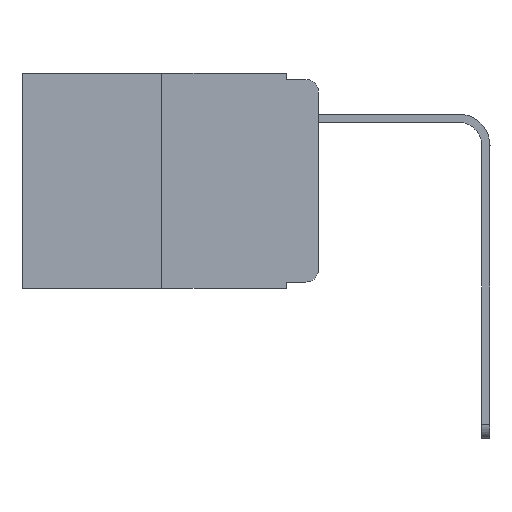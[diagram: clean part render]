
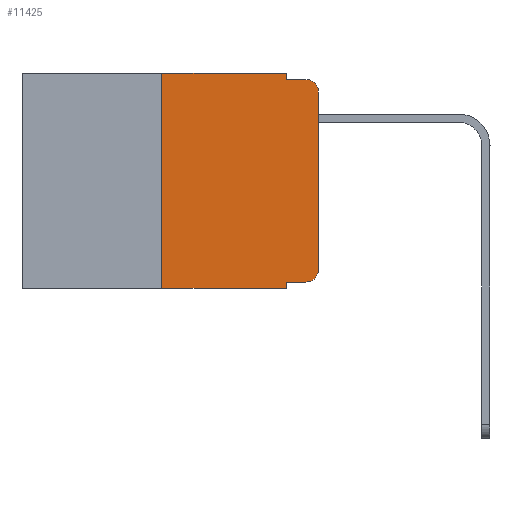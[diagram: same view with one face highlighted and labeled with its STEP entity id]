
A CAD part, left-side view. The second image highlights one B-rep face of the part: STEP entity #11425.
In plain terms, the highlighted planar face has unit normal (-1, 0, 0).
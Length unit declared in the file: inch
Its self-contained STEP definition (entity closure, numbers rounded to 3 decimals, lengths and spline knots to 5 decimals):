
#719 = VECTOR ( 'NONE', #6921, 39.37008 ) ;
#738 = CIRCLE ( 'NONE', #8596, 0.02 ) ;
#768 = DIRECTION ( 'NONE',  ( 1., 0., 0. ) ) ;
#1142 = CARTESIAN_POINT ( 'NONE',  ( 0., 0.051, -0.333 ) ) ;
#1463 = CARTESIAN_POINT ( 'NONE',  ( 0., 0.051, 0. ) ) ;
#1573 = VECTOR ( 'NONE', #10688, 39.37008 ) ;
#1905 = ORIENTED_EDGE ( 'NONE', *, *, #14306, .F. ) ;
#2020 = CARTESIAN_POINT ( 'NONE',  ( 0., 0.051, -0.343 ) ) ;
#2275 = LINE ( 'NONE', #13349, #10521 ) ;
#2339 = CARTESIAN_POINT ( 'NONE',  ( 0., 0., 0. ) ) ;
#2434 = EDGE_CURVE ( 'NONE', #6077, #4303, #13875, .T. ) ;
#2493 = DIRECTION ( 'NONE',  ( 0., -1., 0. ) ) ;
#2670 = EDGE_CURVE ( 'NONE', #12390, #6077, #7057, .T. ) ;
#2777 = CARTESIAN_POINT ( 'NONE',  ( 0., 0.25, 0. ) ) ;
#2807 = CARTESIAN_POINT ( 'NONE',  ( 0., 0.25, 0. ) ) ;
#2841 = ORIENTED_EDGE ( 'NONE', *, *, #4128, .T. ) ;
#2845 = EDGE_CURVE ( 'NONE', #5202, #4857, #7710, .T. ) ;
#2945 = ORIENTED_EDGE ( 'NONE', *, *, #12953, .T. ) ;
#3243 = ORIENTED_EDGE ( 'NONE', *, *, #2845, .F. ) ;
#3553 = CIRCLE ( 'NONE', #8118, 0.02 ) ;
#3591 = CARTESIAN_POINT ( 'NONE',  ( 0., 0.473, -0.343 ) ) ;
#3606 = VECTOR ( 'NONE', #11554, 39.37008 ) ;
#3711 = ORIENTED_EDGE ( 'NONE', *, *, #2434, .F. ) ;
#3738 = DIRECTION ( 'NONE',  ( 0., -1., 0. ) ) ;
#3807 = VERTEX_POINT ( 'NONE', #2020 ) ;
#3950 = VERTEX_POINT ( 'NONE', #11435 ) ;
#4086 = VECTOR ( 'NONE', #3738, 39.37008 ) ;
#4126 = CARTESIAN_POINT ( 'NONE',  ( 0., 0.473, 0. ) ) ;
#4128 = EDGE_CURVE ( 'NONE', #10105, #5263, #7349, .T. ) ;
#4303 = VERTEX_POINT ( 'NONE', #12466 ) ;
#4337 = CARTESIAN_POINT ( 'NONE',  ( 0., 0.02, -0.03 ) ) ;
#4547 = ORIENTED_EDGE ( 'NONE', *, *, #9594, .T. ) ;
#4581 = CARTESIAN_POINT ( 'NONE',  ( 0., 0.051, -0.01 ) ) ;
#4683 = DIRECTION ( 'NONE',  ( 0., -1., 0. ) ) ;
#4857 = VERTEX_POINT ( 'NONE', #2777 ) ;
#5202 = VERTEX_POINT ( 'NONE', #13880 ) ;
#5263 = VERTEX_POINT ( 'NONE', #11961 ) ;
#5633 = ORIENTED_EDGE ( 'NONE', *, *, #11027, .T. ) ;
#6077 = VERTEX_POINT ( 'NONE', #4581 ) ;
#6212 = LINE ( 'NONE', #3591, #7928 ) ;
#6633 = DIRECTION ( 'NONE',  ( 0., 0., -1. ) ) ;
#6648 = CARTESIAN_POINT ( 'NONE',  ( 0., 0.051, -0.333 ) ) ;
#6921 = DIRECTION ( 'NONE',  ( 0., 0., -1. ) ) ;
#7057 = LINE ( 'NONE', #12367, #719 ) ;
#7072 = VECTOR ( 'NONE', #2493, 39.37008 ) ;
#7349 = LINE ( 'NONE', #1142, #10670 ) ;
#7529 = ORIENTED_EDGE ( 'NONE', *, *, #13094, .F. ) ;
#7585 = DIRECTION ( 'NONE',  ( 0., 0., -1. ) ) ;
#7710 = LINE ( 'NONE', #2807, #1573 ) ;
#7928 = VECTOR ( 'NONE', #4683, 39.37008 ) ;
#8118 = AXIS2_PLACEMENT_3D ( 'NONE', #4337, #12115, #7585 ) ;
#8596 = AXIS2_PLACEMENT_3D ( 'NONE', #12585, #13663, #11418 ) ;
#9594 = EDGE_CURVE ( 'NONE', #11531, #3950, #9907, .T. ) ;
#9907 = LINE ( 'NONE', #2339, #3606 ) ;
#9993 = EDGE_LOOP ( 'NONE', ( #4547, #5633, #3711, #12923, #7529, #3243, #2945, #1905, #2841, #13363 ) ) ;
#10105 = VERTEX_POINT ( 'NONE', #6648 ) ;
#10115 = AXIS2_PLACEMENT_3D ( 'NONE', #4126, #768, #14008 ) ;
#10212 = DIRECTION ( 'NONE',  ( 0., -1., 0. ) ) ;
#10442 = CARTESIAN_POINT ( 'NONE',  ( 0., 0.051, -0.01 ) ) ;
#10521 = VECTOR ( 'NONE', #6633, 39.37008 ) ;
#10619 = PLANE ( 'NONE',  #10115 ) ;
#10670 = VECTOR ( 'NONE', #10212, 39.37008 ) ;
#10688 = DIRECTION ( 'NONE',  ( 0., 0., 1. ) ) ;
#10802 = EDGE_CURVE ( 'NONE', #5263, #11531, #738, .T. ) ;
#11027 = EDGE_CURVE ( 'NONE', #3950, #4303, #3553, .T. ) ;
#11417 = FACE_OUTER_BOUND ( 'NONE', #9993, .T. ) ;
#11418 = DIRECTION ( 'NONE',  ( 0., 0., -1. ) ) ;
#11425 = ADVANCED_FACE ( 'NONE', ( #11417 ), #10619, .F. ) ;
#11435 = CARTESIAN_POINT ( 'NONE',  ( 0., 0., -0.03 ) ) ;
#11531 = VERTEX_POINT ( 'NONE', #12919 ) ;
#11554 = DIRECTION ( 'NONE',  ( 0., 0., 1. ) ) ;
#11961 = CARTESIAN_POINT ( 'NONE',  ( 0., 0.02, -0.333 ) ) ;
#12115 = DIRECTION ( 'NONE',  ( -1., 0., 0. ) ) ;
#12367 = CARTESIAN_POINT ( 'NONE',  ( 0., 0.051, 0. ) ) ;
#12390 = VERTEX_POINT ( 'NONE', #1463 ) ;
#12466 = CARTESIAN_POINT ( 'NONE',  ( 0., 0.02, -0.01 ) ) ;
#12585 = CARTESIAN_POINT ( 'NONE',  ( 0., 0.02, -0.313 ) ) ;
#12779 = CARTESIAN_POINT ( 'NONE',  ( 0., 0.473, 0. ) ) ;
#12919 = CARTESIAN_POINT ( 'NONE',  ( 0., 0., -0.313 ) ) ;
#12923 = ORIENTED_EDGE ( 'NONE', *, *, #2670, .F. ) ;
#12953 = EDGE_CURVE ( 'NONE', #5202, #3807, #6212, .T. ) ;
#13094 = EDGE_CURVE ( 'NONE', #4857, #12390, #13530, .T. ) ;
#13349 = CARTESIAN_POINT ( 'NONE',  ( 0., 0.051, 0. ) ) ;
#13363 = ORIENTED_EDGE ( 'NONE', *, *, #10802, .T. ) ;
#13530 = LINE ( 'NONE', #12779, #7072 ) ;
#13663 = DIRECTION ( 'NONE',  ( -1., 0., 0. ) ) ;
#13875 = LINE ( 'NONE', #10442, #4086 ) ;
#13880 = CARTESIAN_POINT ( 'NONE',  ( 0., 0.25, -0.343 ) ) ;
#14008 = DIRECTION ( 'NONE',  ( 0., 0., -1. ) ) ;
#14306 = EDGE_CURVE ( 'NONE', #10105, #3807, #2275, .T. ) ;
